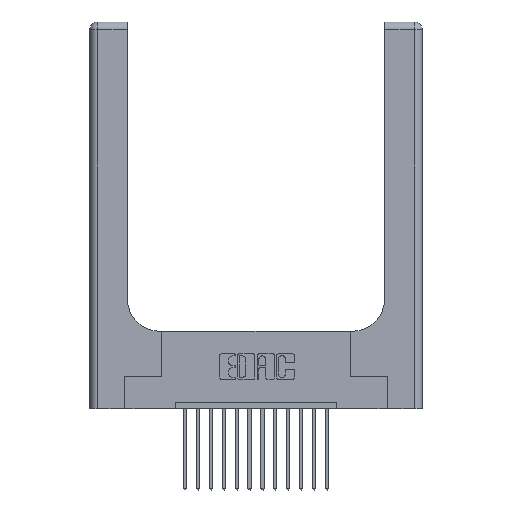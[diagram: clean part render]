
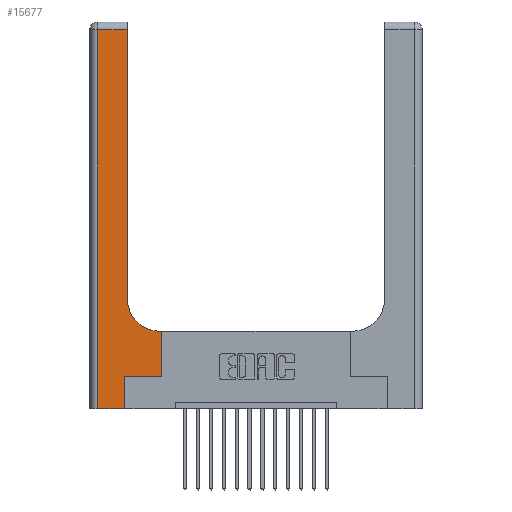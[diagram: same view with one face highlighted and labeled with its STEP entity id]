
A CAD part, top view. The second image highlights one B-rep face of the part: STEP entity #15677.
In plain terms, the highlighted planar face has unit normal (0, 0, 1).
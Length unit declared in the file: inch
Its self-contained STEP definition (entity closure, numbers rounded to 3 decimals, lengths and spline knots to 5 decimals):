
#161 = DIRECTION ( 'NONE',  ( 0., 1., 0. ) ) ;
#238 = VECTOR ( 'NONE', #6897, 39.37008 ) ;
#458 = ORIENTED_EDGE ( 'NONE', *, *, #17523, .T. ) ;
#765 = VERTEX_POINT ( 'NONE', #3711 ) ;
#1148 = ORIENTED_EDGE ( 'NONE', *, *, #9249, .T. ) ;
#1174 = LINE ( 'NONE', #1590, #11545 ) ;
#1288 = ORIENTED_EDGE ( 'NONE', *, *, #3905, .T. ) ;
#1292 = VECTOR ( 'NONE', #161, 39.37008 ) ;
#1523 = CARTESIAN_POINT ( 'NONE',  ( 0.5585, 0.25, 0.37 ) ) ;
#1590 = CARTESIAN_POINT ( 'NONE',  ( 0.2915, 0.6, 0.37 ) ) ;
#1737 = CARTESIAN_POINT ( 'NONE',  ( 0.06, 0., 0.37 ) ) ;
#1857 = DIRECTION ( 'NONE',  ( -1., 0., 0. ) ) ;
#1919 = CARTESIAN_POINT ( 'NONE',  ( 0., 3., 0.37 ) ) ;
#2045 = LINE ( 'NONE', #7822, #16634 ) ;
#2062 = AXIS2_PLACEMENT_3D ( 'NONE', #1919, #4636, #1857 ) ;
#2264 = DIRECTION ( 'NONE',  ( -1., 0., 0. ) ) ;
#3107 = EDGE_LOOP ( 'NONE', ( #14875, #458, #16848, #15789, #1148, #5695, #1288, #12128, #12271 ) ) ;
#3502 = LINE ( 'NONE', #5764, #1292 ) ;
#3677 = VECTOR ( 'NONE', #2264, 39.37008 ) ;
#3711 = CARTESIAN_POINT ( 'NONE',  ( 0.269, 0.25, 0.37 ) ) ;
#3905 = EDGE_CURVE ( 'NONE', #9946, #10462, #3502, .T. ) ;
#4104 = EDGE_CURVE ( 'NONE', #14021, #12922, #4603, .T. ) ;
#4603 = LINE ( 'NONE', #17829, #11005 ) ;
#4636 = DIRECTION ( 'NONE',  ( 0., 0., -1. ) ) ;
#5330 = VECTOR ( 'NONE', #9179, 39.37008 ) ;
#5659 = VERTEX_POINT ( 'NONE', #12007 ) ;
#5695 = ORIENTED_EDGE ( 'NONE', *, *, #7899, .T. ) ;
#5764 = CARTESIAN_POINT ( 'NONE',  ( 0.5585, 0.25, 0.37 ) ) ;
#6645 = LINE ( 'NONE', #14309, #5330 ) ;
#6897 = DIRECTION ( 'NONE',  ( 0., 1., 0. ) ) ;
#7290 = VECTOR ( 'NONE', #9280, 39.37008 ) ;
#7520 = LINE ( 'NONE', #7615, #7290 ) ;
#7549 = FACE_OUTER_BOUND ( 'NONE', #3107, .T. ) ;
#7615 = CARTESIAN_POINT ( 'NONE',  ( 0.06, 3., 0.37 ) ) ;
#7667 = CARTESIAN_POINT ( 'NONE',  ( 0.5415, 0.6, 0.37 ) ) ;
#7758 = VERTEX_POINT ( 'NONE', #15613 ) ;
#7822 = CARTESIAN_POINT ( 'NONE',  ( 0.269, 0.25, 0.37 ) ) ;
#7899 = EDGE_CURVE ( 'NONE', #765, #9946, #2045, .T. ) ;
#8255 = CARTESIAN_POINT ( 'NONE',  ( 0.5415, 0.85, 0.37 ) ) ;
#9179 = DIRECTION ( 'NONE',  ( 1., 0., 0. ) ) ;
#9249 = EDGE_CURVE ( 'NONE', #7758, #765, #11267, .T. ) ;
#9280 = DIRECTION ( 'NONE',  ( 0., -1., 0. ) ) ;
#9789 = EDGE_CURVE ( 'NONE', #5659, #18008, #7520, .T. ) ;
#9946 = VERTEX_POINT ( 'NONE', #1523 ) ;
#9955 = CARTESIAN_POINT ( 'NONE',  ( 0.2915, 0.85, 0.37 ) ) ;
#10251 = CIRCLE ( 'NONE', #14488, 0.25 ) ;
#10273 = EDGE_CURVE ( 'NONE', #18008, #7758, #6645, .T. ) ;
#10462 = VERTEX_POINT ( 'NONE', #14476 ) ;
#11005 = VECTOR ( 'NONE', #12086, 39.37008 ) ;
#11267 = LINE ( 'NONE', #12273, #238 ) ;
#11434 = DIRECTION ( 'NONE',  ( -1., 0., 0. ) ) ;
#11545 = VECTOR ( 'NONE', #11434, 39.37008 ) ;
#11610 = LINE ( 'NONE', #16586, #3677 ) ;
#12007 = CARTESIAN_POINT ( 'NONE',  ( 0.06, 2.94, 0.37 ) ) ;
#12086 = DIRECTION ( 'NONE',  ( 0., 1., 0. ) ) ;
#12128 = ORIENTED_EDGE ( 'NONE', *, *, #15919, .T. ) ;
#12271 = ORIENTED_EDGE ( 'NONE', *, *, #17741, .T. ) ;
#12273 = CARTESIAN_POINT ( 'NONE',  ( 0.269, 0., 0.37 ) ) ;
#12500 = DIRECTION ( 'NONE',  ( 0., 0., -1. ) ) ;
#12922 = VERTEX_POINT ( 'NONE', #15299 ) ;
#13136 = PLANE ( 'NONE',  #2062 ) ;
#14021 = VERTEX_POINT ( 'NONE', #9955 ) ;
#14309 = CARTESIAN_POINT ( 'NONE',  ( 0., 0., 0.37 ) ) ;
#14476 = CARTESIAN_POINT ( 'NONE',  ( 0.5585, 0.6, 0.37 ) ) ;
#14488 = AXIS2_PLACEMENT_3D ( 'NONE', #8255, #12500, #18173 ) ;
#14875 = ORIENTED_EDGE ( 'NONE', *, *, #4104, .T. ) ;
#15070 = VERTEX_POINT ( 'NONE', #7667 ) ;
#15299 = CARTESIAN_POINT ( 'NONE',  ( 0.2915, 2.94, 0.37 ) ) ;
#15613 = CARTESIAN_POINT ( 'NONE',  ( 0.269, 0., 0.37 ) ) ;
#15677 = ADVANCED_FACE ( 'NONE', ( #7549 ), #13136, .F. ) ;
#15789 = ORIENTED_EDGE ( 'NONE', *, *, #10273, .T. ) ;
#15919 = EDGE_CURVE ( 'NONE', #10462, #15070, #1174, .T. ) ;
#16586 = CARTESIAN_POINT ( 'NONE',  ( 0., 2.94, 0.37 ) ) ;
#16634 = VECTOR ( 'NONE', #17842, 39.37008 ) ;
#16848 = ORIENTED_EDGE ( 'NONE', *, *, #9789, .T. ) ;
#17523 = EDGE_CURVE ( 'NONE', #12922, #5659, #11610, .T. ) ;
#17741 = EDGE_CURVE ( 'NONE', #15070, #14021, #10251, .T. ) ;
#17829 = CARTESIAN_POINT ( 'NONE',  ( 0.2915, 3., 0.37 ) ) ;
#17842 = DIRECTION ( 'NONE',  ( 1., 0., 0. ) ) ;
#18008 = VERTEX_POINT ( 'NONE', #1737 ) ;
#18173 = DIRECTION ( 'NONE',  ( 1., 0., 0. ) ) ;
